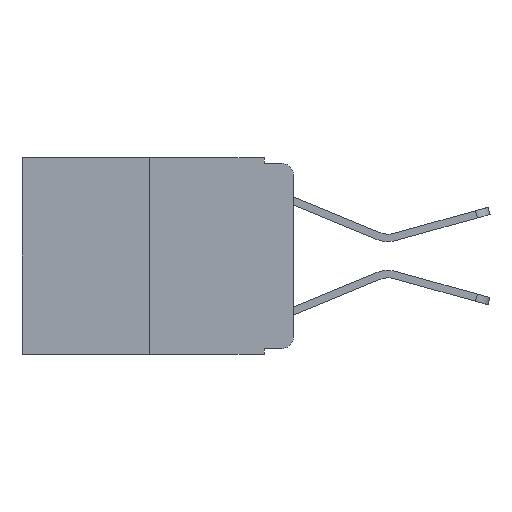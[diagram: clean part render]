
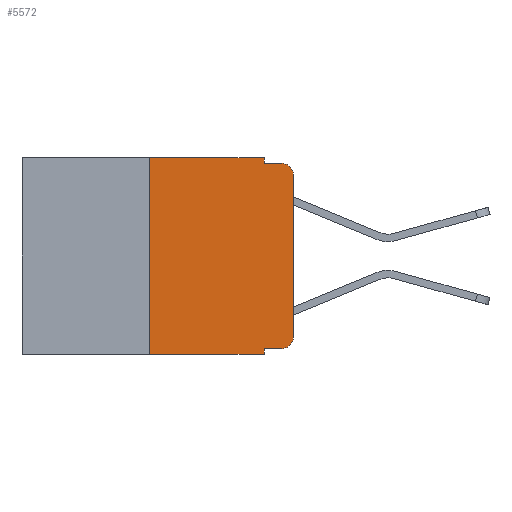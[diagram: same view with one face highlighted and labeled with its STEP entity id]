
A CAD part, left-side view. The second image highlights one B-rep face of the part: STEP entity #5572.
In plain terms, the highlighted planar face has unit normal (-1, 0, 0).
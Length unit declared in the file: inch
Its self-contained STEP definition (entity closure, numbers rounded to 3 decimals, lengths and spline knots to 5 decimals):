
#313 = DIRECTION ( 'NONE',  ( 0., 0., -1. ) ) ;
#327 = VECTOR ( 'NONE', #14450, 39.37008 ) ;
#407 = EDGE_CURVE ( 'NONE', #8257, #4272, #3550, .T. ) ;
#557 = EDGE_CURVE ( 'NONE', #8257, #16021, #9964, .T. ) ;
#684 = VERTEX_POINT ( 'NONE', #12447 ) ;
#740 = VECTOR ( 'NONE', #7476, 39.37008 ) ;
#756 = FACE_OUTER_BOUND ( 'NONE', #2158, .T. ) ;
#818 = ORIENTED_EDGE ( 'NONE', *, *, #6815, .F. ) ;
#915 = EDGE_CURVE ( 'NONE', #10126, #16021, #15702, .T. ) ;
#1033 = VECTOR ( 'NONE', #8728, 39.37008 ) ;
#1157 = DIRECTION ( 'NONE',  ( -1., 0., 0. ) ) ;
#1200 = CARTESIAN_POINT ( 'NONE',  ( 0., 0.02, -0.01 ) ) ;
#1426 = LINE ( 'NONE', #10413, #6340 ) ;
#1476 = CARTESIAN_POINT ( 'NONE',  ( 0., 0.051, -0.333 ) ) ;
#1889 = DIRECTION ( 'NONE',  ( 0., -1., 0. ) ) ;
#1974 = LINE ( 'NONE', #5620, #10668 ) ;
#2158 = EDGE_LOOP ( 'NONE', ( #7826, #11978, #4221, #7405, #14126, #818, #15121, #11170, #13618, #8681 ) ) ;
#2193 = CARTESIAN_POINT ( 'NONE',  ( 0., 0.25, 0. ) ) ;
#2392 = CARTESIAN_POINT ( 'NONE',  ( 0., 0.051, 0. ) ) ;
#2496 = CARTESIAN_POINT ( 'NONE',  ( 0., 0., -0.313 ) ) ;
#2597 = DIRECTION ( 'NONE',  ( 0., 0., 1. ) ) ;
#2610 = CARTESIAN_POINT ( 'NONE',  ( 0., 0., -0.03 ) ) ;
#2909 = EDGE_CURVE ( 'NONE', #6703, #15981, #1974, .T. ) ;
#3312 = DIRECTION ( 'NONE',  ( 1., 0., 0. ) ) ;
#3550 = LINE ( 'NONE', #1476, #740 ) ;
#4221 = ORIENTED_EDGE ( 'NONE', *, *, #13212, .F. ) ;
#4272 = VERTEX_POINT ( 'NONE', #7138 ) ;
#4289 = CARTESIAN_POINT ( 'NONE',  ( 0., 0.473, -0.343 ) ) ;
#4904 = CARTESIAN_POINT ( 'NONE',  ( 0., 0.051, 0. ) ) ;
#5158 = CARTESIAN_POINT ( 'NONE',  ( 0., 0.25, 0. ) ) ;
#5572 = ADVANCED_FACE ( 'NONE', ( #756 ), #5812, .F. ) ;
#5620 = CARTESIAN_POINT ( 'NONE',  ( 0., 0.473, 0. ) ) ;
#5727 = VERTEX_POINT ( 'NONE', #2496 ) ;
#5812 = PLANE ( 'NONE',  #15732 ) ;
#6163 = EDGE_CURVE ( 'NONE', #13719, #9757, #15842, .T. ) ;
#6203 = DIRECTION ( 'NONE',  ( 0., 0., -1. ) ) ;
#6340 = VECTOR ( 'NONE', #2597, 39.37008 ) ;
#6472 = EDGE_CURVE ( 'NONE', #4272, #5727, #16174, .T. ) ;
#6680 = CARTESIAN_POINT ( 'NONE',  ( 0., 0.051, -0.333 ) ) ;
#6703 = VERTEX_POINT ( 'NONE', #2193 ) ;
#6815 = EDGE_CURVE ( 'NONE', #10126, #6703, #10257, .T. ) ;
#7138 = CARTESIAN_POINT ( 'NONE',  ( 0., 0.02, -0.333 ) ) ;
#7303 = DIRECTION ( 'NONE',  ( 0., 0., -1. ) ) ;
#7405 = ORIENTED_EDGE ( 'NONE', *, *, #14040, .F. ) ;
#7476 = DIRECTION ( 'NONE',  ( 0., -1., 0. ) ) ;
#7826 = ORIENTED_EDGE ( 'NONE', *, *, #15906, .T. ) ;
#7850 = DIRECTION ( 'NONE',  ( -1., 0., 0. ) ) ;
#8257 = VERTEX_POINT ( 'NONE', #6680 ) ;
#8674 = CARTESIAN_POINT ( 'NONE',  ( 0., 0.25, -0.343 ) ) ;
#8681 = ORIENTED_EDGE ( 'NONE', *, *, #6472, .T. ) ;
#8728 = DIRECTION ( 'NONE',  ( 0., 0., -1. ) ) ;
#8822 = CARTESIAN_POINT ( 'NONE',  ( 0., 0.051, -0.01 ) ) ;
#8916 = DIRECTION ( 'NONE',  ( 0., 0., -1. ) ) ;
#9012 = AXIS2_PLACEMENT_3D ( 'NONE', #15280, #7850, #313 ) ;
#9757 = VERTEX_POINT ( 'NONE', #1200 ) ;
#9813 = VECTOR ( 'NONE', #8916, 39.37008 ) ;
#9964 = LINE ( 'NONE', #2392, #1033 ) ;
#10126 = VERTEX_POINT ( 'NONE', #8674 ) ;
#10257 = LINE ( 'NONE', #5158, #12268 ) ;
#10413 = CARTESIAN_POINT ( 'NONE',  ( 0., 0., 0. ) ) ;
#10668 = VECTOR ( 'NONE', #1889, 39.37008 ) ;
#10812 = AXIS2_PLACEMENT_3D ( 'NONE', #12557, #1157, #6203 ) ;
#11170 = ORIENTED_EDGE ( 'NONE', *, *, #557, .F. ) ;
#11172 = CARTESIAN_POINT ( 'NONE',  ( 0., 0.473, 0. ) ) ;
#11368 = DIRECTION ( 'NONE',  ( 0., 0., 1. ) ) ;
#11467 = DIRECTION ( 'NONE',  ( 0., -1., 0. ) ) ;
#11517 = CARTESIAN_POINT ( 'NONE',  ( 0., 0.051, -0.343 ) ) ;
#11585 = CARTESIAN_POINT ( 'NONE',  ( 0., 0.051, 0. ) ) ;
#11978 = ORIENTED_EDGE ( 'NONE', *, *, #6163, .T. ) ;
#12268 = VECTOR ( 'NONE', #11368, 39.37008 ) ;
#12447 = CARTESIAN_POINT ( 'NONE',  ( 0., 0.051, -0.01 ) ) ;
#12557 = CARTESIAN_POINT ( 'NONE',  ( 0., 0.02, -0.03 ) ) ;
#12743 = LINE ( 'NONE', #4904, #9813 ) ;
#13212 = EDGE_CURVE ( 'NONE', #684, #9757, #13789, .T. ) ;
#13618 = ORIENTED_EDGE ( 'NONE', *, *, #407, .T. ) ;
#13719 = VERTEX_POINT ( 'NONE', #2610 ) ;
#13789 = LINE ( 'NONE', #8822, #16160 ) ;
#14040 = EDGE_CURVE ( 'NONE', #15981, #684, #12743, .T. ) ;
#14126 = ORIENTED_EDGE ( 'NONE', *, *, #2909, .F. ) ;
#14450 = DIRECTION ( 'NONE',  ( 0., -1., 0. ) ) ;
#15121 = ORIENTED_EDGE ( 'NONE', *, *, #915, .T. ) ;
#15280 = CARTESIAN_POINT ( 'NONE',  ( 0., 0.02, -0.313 ) ) ;
#15702 = LINE ( 'NONE', #4289, #327 ) ;
#15732 = AXIS2_PLACEMENT_3D ( 'NONE', #11172, #3312, #7303 ) ;
#15842 = CIRCLE ( 'NONE', #10812, 0.02 ) ;
#15906 = EDGE_CURVE ( 'NONE', #5727, #13719, #1426, .T. ) ;
#15981 = VERTEX_POINT ( 'NONE', #11585 ) ;
#16021 = VERTEX_POINT ( 'NONE', #11517 ) ;
#16160 = VECTOR ( 'NONE', #11467, 39.37008 ) ;
#16174 = CIRCLE ( 'NONE', #9012, 0.02 ) ;
